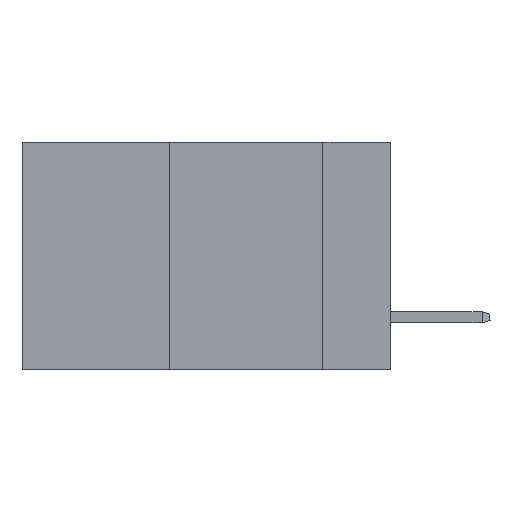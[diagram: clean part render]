
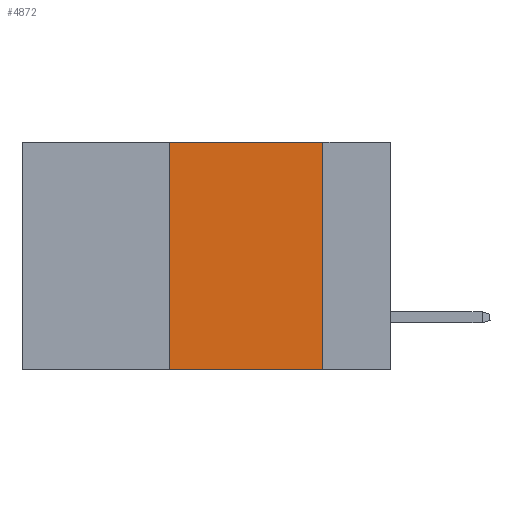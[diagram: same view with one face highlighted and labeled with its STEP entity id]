
A CAD part, left-side view. The second image highlights one B-rep face of the part: STEP entity #4872.
In plain terms, the highlighted planar face has unit normal (-1, 0, 0).
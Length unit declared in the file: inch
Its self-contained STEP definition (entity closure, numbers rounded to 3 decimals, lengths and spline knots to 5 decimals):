
#124 = DIRECTION ( 'NONE',  ( 1., 0., 0. ) ) ;
#488 = LINE ( 'NONE', #5695, #6658 ) ;
#611 = ORIENTED_EDGE ( 'NONE', *, *, #3281, .F. ) ;
#1592 = CARTESIAN_POINT ( 'NONE',  ( 0., 0.11, 0. ) ) ;
#2032 = VECTOR ( 'NONE', #10877, 39.37008 ) ;
#2211 = EDGE_LOOP ( 'NONE', ( #4007, #611, #3183, #7953 ) ) ;
#2344 = FACE_OUTER_BOUND ( 'NONE', #2211, .T. ) ;
#2409 = CARTESIAN_POINT ( 'NONE',  ( 0., 0.6, 0. ) ) ;
#2929 = LINE ( 'NONE', #8485, #2032 ) ;
#3183 = ORIENTED_EDGE ( 'NONE', *, *, #6739, .F. ) ;
#3281 = EDGE_CURVE ( 'NONE', #12028, #6756, #2929, .T. ) ;
#3458 = DIRECTION ( 'NONE',  ( 0., 0., -1. ) ) ;
#4007 = ORIENTED_EDGE ( 'NONE', *, *, #10911, .F. ) ;
#4872 = ADVANCED_FACE ( 'NONE', ( #2344 ), #8264, .F. ) ;
#5147 = CARTESIAN_POINT ( 'NONE',  ( 0., 0.11, 0. ) ) ;
#5695 = CARTESIAN_POINT ( 'NONE',  ( 0., 0.36, 0. ) ) ;
#6658 = VECTOR ( 'NONE', #6934, 39.37008 ) ;
#6739 = EDGE_CURVE ( 'NONE', #11556, #12028, #488, .T. ) ;
#6756 = VERTEX_POINT ( 'NONE', #5147 ) ;
#6891 = VECTOR ( 'NONE', #7084, 39.37008 ) ;
#6934 = DIRECTION ( 'NONE',  ( 0., 0., 1. ) ) ;
#7084 = DIRECTION ( 'NONE',  ( 0., -1., 0. ) ) ;
#7113 = CARTESIAN_POINT ( 'NONE',  ( 0., 0.11, -0.37 ) ) ;
#7953 = ORIENTED_EDGE ( 'NONE', *, *, #8630, .T. ) ;
#8214 = CARTESIAN_POINT ( 'NONE',  ( 0., 0.36, -0.37 ) ) ;
#8264 = PLANE ( 'NONE',  #12505 ) ;
#8485 = CARTESIAN_POINT ( 'NONE',  ( 0., 0.6, 0. ) ) ;
#8630 = EDGE_CURVE ( 'NONE', #11556, #14581, #10539, .T. ) ;
#9609 = DIRECTION ( 'NONE',  ( 0., 0., -1. ) ) ;
#10539 = LINE ( 'NONE', #12800, #6891 ) ;
#10578 = CARTESIAN_POINT ( 'NONE',  ( 0., 0.36, 0. ) ) ;
#10877 = DIRECTION ( 'NONE',  ( 0., -1., 0. ) ) ;
#10911 = EDGE_CURVE ( 'NONE', #6756, #14581, #11375, .T. ) ;
#11034 = VECTOR ( 'NONE', #9609, 39.37008 ) ;
#11375 = LINE ( 'NONE', #1592, #11034 ) ;
#11556 = VERTEX_POINT ( 'NONE', #8214 ) ;
#12028 = VERTEX_POINT ( 'NONE', #10578 ) ;
#12505 = AXIS2_PLACEMENT_3D ( 'NONE', #2409, #124, #3458 ) ;
#12800 = CARTESIAN_POINT ( 'NONE',  ( 0., 0.6, -0.37 ) ) ;
#14581 = VERTEX_POINT ( 'NONE', #7113 ) ;
